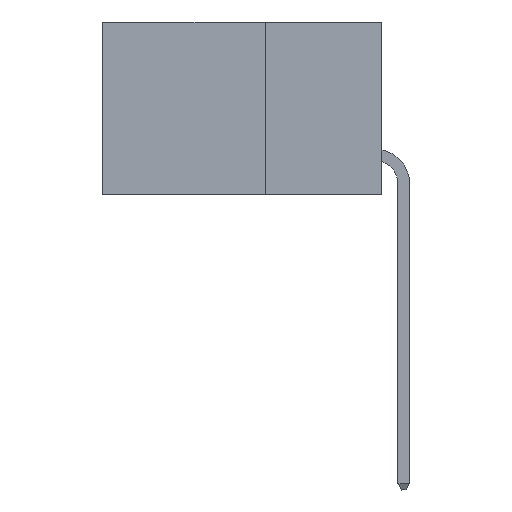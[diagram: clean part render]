
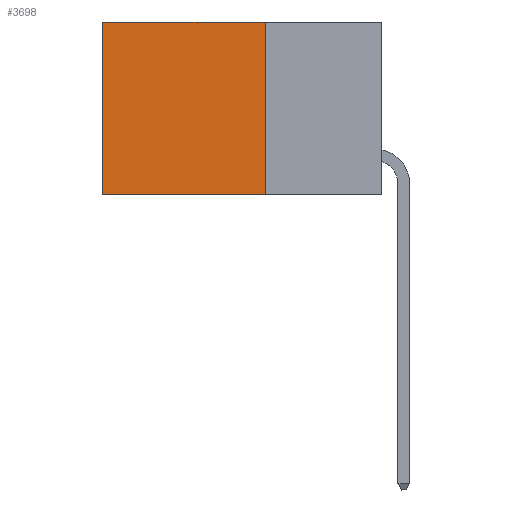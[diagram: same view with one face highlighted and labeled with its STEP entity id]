
A CAD part, left-side view. The second image highlights one B-rep face of the part: STEP entity #3698.
In plain terms, the highlighted planar face has unit normal (-1, 0, 0).
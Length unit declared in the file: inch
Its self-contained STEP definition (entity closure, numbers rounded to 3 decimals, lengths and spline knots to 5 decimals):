
#233 = AXIS2_PLACEMENT_3D ( 'NONE', #24424, #5226, #20942 ) ;
#1256 = CARTESIAN_POINT ( 'NONE',  ( 0.2875, 0.25, 0. ) ) ;
#1409 = PLANE ( 'NONE',  #233 ) ;
#2286 = CARTESIAN_POINT ( 'NONE',  ( 0.2875, 0.6, 0. ) ) ;
#2630 = EDGE_CURVE ( 'NONE', #14107, #5283, #12669, .T. ) ;
#3698 = ADVANCED_FACE ( 'NONE', ( #27597 ), #1409, .F. ) ;
#4126 = VECTOR ( 'NONE', #22616, 39.37008 ) ;
#4552 = ORIENTED_EDGE ( 'NONE', *, *, #9008, .F. ) ;
#5226 = DIRECTION ( 'NONE',  ( 1., 0., 0. ) ) ;
#5283 = VERTEX_POINT ( 'NONE', #12453 ) ;
#8133 = EDGE_CURVE ( 'NONE', #25055, #5283, #36005, .T. ) ;
#9008 = EDGE_CURVE ( 'NONE', #17648, #25055, #23346, .T. ) ;
#12453 = CARTESIAN_POINT ( 'NONE',  ( 0.2875, 0.6, -0.37 ) ) ;
#12669 = LINE ( 'NONE', #2286, #4126 ) ;
#13941 = VECTOR ( 'NONE', #32417, 39.37008 ) ;
#14107 = VERTEX_POINT ( 'NONE', #21135 ) ;
#14997 = ORIENTED_EDGE ( 'NONE', *, *, #8133, .F. ) ;
#16989 = EDGE_CURVE ( 'NONE', #17648, #14107, #23732, .T. ) ;
#17068 = DIRECTION ( 'NONE',  ( 0., 1., 0. ) ) ;
#17648 = VERTEX_POINT ( 'NONE', #1256 ) ;
#18205 = EDGE_LOOP ( 'NONE', ( #39456, #14997, #4552, #33864 ) ) ;
#20838 = VECTOR ( 'NONE', #34151, 39.37008 ) ;
#20942 = DIRECTION ( 'NONE',  ( 0., 0., -1. ) ) ;
#20973 = CARTESIAN_POINT ( 'NONE',  ( 0.2875, 0.25, 0. ) ) ;
#21135 = CARTESIAN_POINT ( 'NONE',  ( 0.2875, 0.6, 0. ) ) ;
#22616 = DIRECTION ( 'NONE',  ( 0., 0., -1. ) ) ;
#23346 = LINE ( 'NONE', #20973, #20838 ) ;
#23732 = LINE ( 'NONE', #27015, #34750 ) ;
#24424 = CARTESIAN_POINT ( 'NONE',  ( 0.2875, 0.25, 0. ) ) ;
#25055 = VERTEX_POINT ( 'NONE', #31343 ) ;
#27015 = CARTESIAN_POINT ( 'NONE',  ( 0.2875, 0.25, 0. ) ) ;
#27597 = FACE_OUTER_BOUND ( 'NONE', #18205, .T. ) ;
#31343 = CARTESIAN_POINT ( 'NONE',  ( 0.2875, 0.25, -0.37 ) ) ;
#32417 = DIRECTION ( 'NONE',  ( 0., 1., 0. ) ) ;
#32694 = CARTESIAN_POINT ( 'NONE',  ( 0.2875, 0.25, -0.37 ) ) ;
#33864 = ORIENTED_EDGE ( 'NONE', *, *, #16989, .T. ) ;
#34151 = DIRECTION ( 'NONE',  ( 0., 0., -1. ) ) ;
#34750 = VECTOR ( 'NONE', #17068, 39.37008 ) ;
#36005 = LINE ( 'NONE', #32694, #13941 ) ;
#39456 = ORIENTED_EDGE ( 'NONE', *, *, #2630, .T. ) ;
